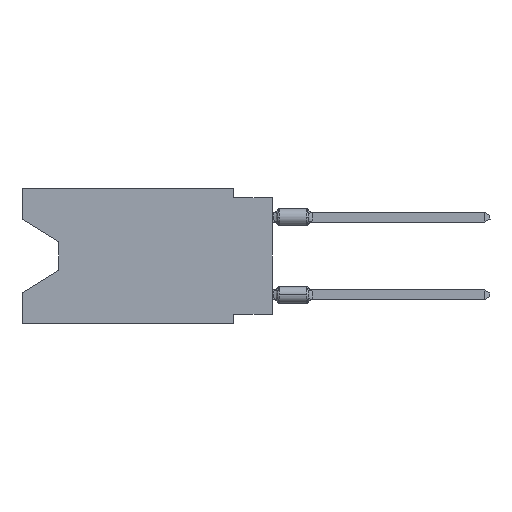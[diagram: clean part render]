
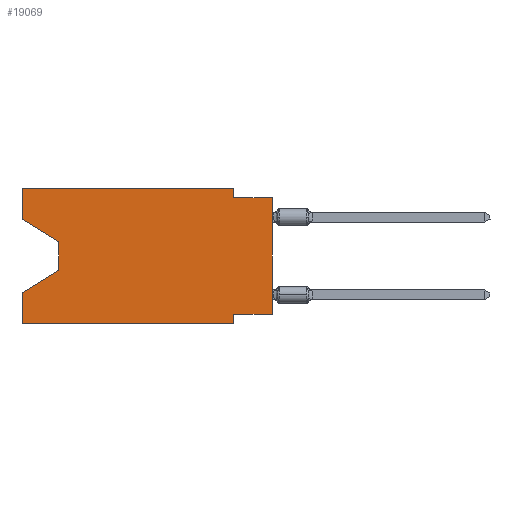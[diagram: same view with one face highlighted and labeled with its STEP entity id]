
A CAD part, left-side view. The second image highlights one B-rep face of the part: STEP entity #19069.
In plain terms, the highlighted planar face has unit normal (-1, 0, 0).
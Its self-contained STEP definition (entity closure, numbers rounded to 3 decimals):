
#234 = ORIENTED_EDGE ( 'NONE', *, *, #35862, .T. ) ;
#249 = CARTESIAN_POINT ( 'NONE',  ( 0., 0., -8.255 ) ) ;
#677 = FACE_OUTER_BOUND ( 'NONE', #31317, .T. ) ;
#944 = CARTESIAN_POINT ( 'NONE',  ( 0., 16.383, 0. ) ) ;
#998 = EDGE_CURVE ( 'NONE', #29977, #4222, #38963, .T. ) ;
#1681 = ORIENTED_EDGE ( 'NONE', *, *, #54526, .T. ) ;
#2020 = EDGE_CURVE ( 'NONE', #31494, #51857, #19224, .T. ) ;
#2035 = VERTEX_POINT ( 'NONE', #49623 ) ;
#2099 = VECTOR ( 'NONE', #31900, 1000. ) ;
#2511 = DIRECTION ( 'NONE',  ( 0., 0., 1. ) ) ;
#3654 = DIRECTION ( 'NONE',  ( 0., -1., 0. ) ) ;
#3809 = LINE ( 'NONE', #17405, #53562 ) ;
#4222 = VERTEX_POINT ( 'NONE', #28821 ) ;
#4573 = DIRECTION ( 'NONE',  ( 0., 0.855, -0.519 ) ) ;
#4785 = VERTEX_POINT ( 'NONE', #15087 ) ;
#5329 = CARTESIAN_POINT ( 'NONE',  ( 0., 16.383, 0. ) ) ;
#5731 = CARTESIAN_POINT ( 'NONE',  ( 0., 0., -8.255 ) ) ;
#6268 = DIRECTION ( 'NONE',  ( 0., 0., -1. ) ) ;
#6310 = DIRECTION ( 'NONE',  ( 0., 1., 0. ) ) ;
#6559 = CARTESIAN_POINT ( 'NONE',  ( 0., 16.383, 0. ) ) ;
#6609 = LINE ( 'NONE', #5731, #28476 ) ;
#6959 = CARTESIAN_POINT ( 'NONE',  ( 0., 16.383, -8.89 ) ) ;
#7305 = ORIENTED_EDGE ( 'NONE', *, *, #53499, .F. ) ;
#8096 = LINE ( 'NONE', #53547, #52204 ) ;
#9234 = CARTESIAN_POINT ( 'NONE',  ( 0., 16.383, 0. ) ) ;
#9359 = ORIENTED_EDGE ( 'NONE', *, *, #19804, .F. ) ;
#9799 = LINE ( 'NONE', #944, #18382 ) ;
#13227 = VERTEX_POINT ( 'NONE', #249 ) ;
#14525 = ORIENTED_EDGE ( 'NONE', *, *, #58135, .T. ) ;
#14762 = VECTOR ( 'NONE', #18918, 1000. ) ;
#15087 = CARTESIAN_POINT ( 'NONE',  ( 0., 0., -0.635 ) ) ;
#15208 = CARTESIAN_POINT ( 'NONE',  ( 0., 16.383, -6.852 ) ) ;
#16014 = DIRECTION ( 'NONE',  ( 0., 0., -1. ) ) ;
#17109 = EDGE_CURVE ( 'NONE', #21773, #43923, #26161, .T. ) ;
#17405 = CARTESIAN_POINT ( 'NONE',  ( 0., 2.54, 0. ) ) ;
#17579 = ORIENTED_EDGE ( 'NONE', *, *, #17109, .F. ) ;
#17907 = VECTOR ( 'NONE', #16014, 1000. ) ;
#18382 = VECTOR ( 'NONE', #20130, 1000. ) ;
#18918 = DIRECTION ( 'NONE',  ( 0., -1., 0. ) ) ;
#19069 = ADVANCED_FACE ( 'NONE', ( #677 ), #46985, .F. ) ;
#19224 = LINE ( 'NONE', #5329, #2099 ) ;
#19804 = EDGE_CURVE ( 'NONE', #43923, #47954, #3809, .T. ) ;
#20130 = DIRECTION ( 'NONE',  ( 0., 0., 1. ) ) ;
#21661 = CARTESIAN_POINT ( 'NONE',  ( 0., 16.383, -2.038 ) ) ;
#21773 = VERTEX_POINT ( 'NONE', #9234 ) ;
#21859 = ORIENTED_EDGE ( 'NONE', *, *, #998, .F. ) ;
#22230 = VECTOR ( 'NONE', #57159, 1000. ) ;
#23520 = CARTESIAN_POINT ( 'NONE',  ( 0., 2.54, -8.255 ) ) ;
#24684 = LINE ( 'NONE', #29961, #43220 ) ;
#24814 = EDGE_CURVE ( 'NONE', #13227, #29977, #6609, .T. ) ;
#26140 = AXIS2_PLACEMENT_3D ( 'NONE', #6559, #36990, #6268 ) ;
#26161 = LINE ( 'NONE', #44149, #22230 ) ;
#26167 = ORIENTED_EDGE ( 'NONE', *, *, #24814, .F. ) ;
#27498 = ORIENTED_EDGE ( 'NONE', *, *, #2020, .F. ) ;
#28476 = VECTOR ( 'NONE', #6310, 1000. ) ;
#28821 = CARTESIAN_POINT ( 'NONE',  ( 0., 2.54, -8.89 ) ) ;
#29482 = CARTESIAN_POINT ( 'NONE',  ( 0., 16.383, -2.038 ) ) ;
#29961 = CARTESIAN_POINT ( 'NONE',  ( 0., 0., 0. ) ) ;
#29977 = VERTEX_POINT ( 'NONE', #23520 ) ;
#31317 = EDGE_LOOP ( 'NONE', ( #1681, #14525, #54507, #27498, #42027, #21859, #26167, #234, #7305, #9359, #17579, #38921 ) ) ;
#31494 = VERTEX_POINT ( 'NONE', #6959 ) ;
#31900 = DIRECTION ( 'NONE',  ( 0., 0., 1. ) ) ;
#34624 = CARTESIAN_POINT ( 'NONE',  ( 0., 2.54, -0.635 ) ) ;
#35538 = CARTESIAN_POINT ( 'NONE',  ( 0., 2.54, 0. ) ) ;
#35862 = EDGE_CURVE ( 'NONE', #13227, #4785, #24684, .T. ) ;
#36617 = CARTESIAN_POINT ( 'NONE',  ( 0., 16.383, -8.89 ) ) ;
#36990 = DIRECTION ( 'NONE',  ( 1., 0., 0. ) ) ;
#38617 = LINE ( 'NONE', #29482, #54158 ) ;
#38921 = ORIENTED_EDGE ( 'NONE', *, *, #39960, .F. ) ;
#38963 = LINE ( 'NONE', #57856, #39771 ) ;
#39134 = CARTESIAN_POINT ( 'NONE',  ( 0., 13.97, -5.385 ) ) ;
#39771 = VECTOR ( 'NONE', #48399, 1000. ) ;
#39960 = EDGE_CURVE ( 'NONE', #49135, #21773, #9799, .T. ) ;
#42027 = ORIENTED_EDGE ( 'NONE', *, *, #42747, .T. ) ;
#42747 = EDGE_CURVE ( 'NONE', #31494, #4222, #45459, .T. ) ;
#43138 = CARTESIAN_POINT ( 'NONE',  ( 0., 13.97, -3.505 ) ) ;
#43220 = VECTOR ( 'NONE', #2511, 1000. ) ;
#43923 = VERTEX_POINT ( 'NONE', #35538 ) ;
#43957 = DIRECTION ( 'NONE',  ( 0., 0., -1. ) ) ;
#44149 = CARTESIAN_POINT ( 'NONE',  ( 0., 16.383, 0. ) ) ;
#44999 = LINE ( 'NONE', #39134, #51745 ) ;
#45459 = LINE ( 'NONE', #36617, #14762 ) ;
#46985 = PLANE ( 'NONE',  #26140 ) ;
#47459 = EDGE_CURVE ( 'NONE', #2035, #51857, #44999, .T. ) ;
#47466 = DIRECTION ( 'NONE',  ( 0., -0.855, -0.519 ) ) ;
#47560 = LINE ( 'NONE', #43138, #17907 ) ;
#47954 = VERTEX_POINT ( 'NONE', #34624 ) ;
#48399 = DIRECTION ( 'NONE',  ( 0., 0., -1. ) ) ;
#49135 = VERTEX_POINT ( 'NONE', #21661 ) ;
#49166 = CARTESIAN_POINT ( 'NONE',  ( 0., 13.97, -3.505 ) ) ;
#49623 = CARTESIAN_POINT ( 'NONE',  ( 0., 13.97, -5.385 ) ) ;
#51745 = VECTOR ( 'NONE', #4573, 1000. ) ;
#51857 = VERTEX_POINT ( 'NONE', #15208 ) ;
#52204 = VECTOR ( 'NONE', #3654, 1000. ) ;
#53499 = EDGE_CURVE ( 'NONE', #47954, #4785, #8096, .T. ) ;
#53547 = CARTESIAN_POINT ( 'NONE',  ( 0., 0., -0.635 ) ) ;
#53562 = VECTOR ( 'NONE', #43957, 1000. ) ;
#54158 = VECTOR ( 'NONE', #47466, 1000. ) ;
#54507 = ORIENTED_EDGE ( 'NONE', *, *, #47459, .T. ) ;
#54526 = EDGE_CURVE ( 'NONE', #49135, #56182, #38617, .T. ) ;
#56182 = VERTEX_POINT ( 'NONE', #49166 ) ;
#57159 = DIRECTION ( 'NONE',  ( 0., -1., 0. ) ) ;
#57856 = CARTESIAN_POINT ( 'NONE',  ( 0., 2.54, -8.89 ) ) ;
#58135 = EDGE_CURVE ( 'NONE', #56182, #2035, #47560, .T. ) ;
